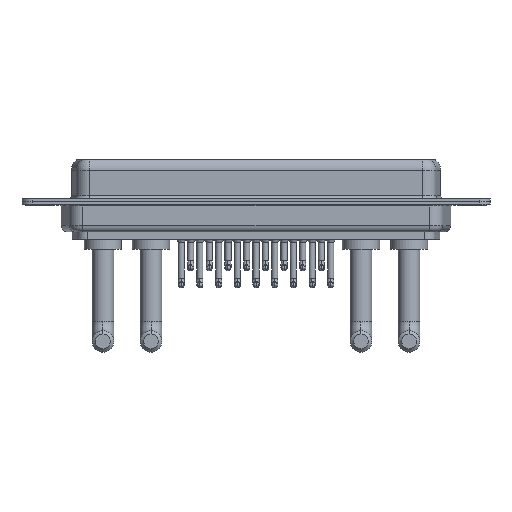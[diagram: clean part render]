
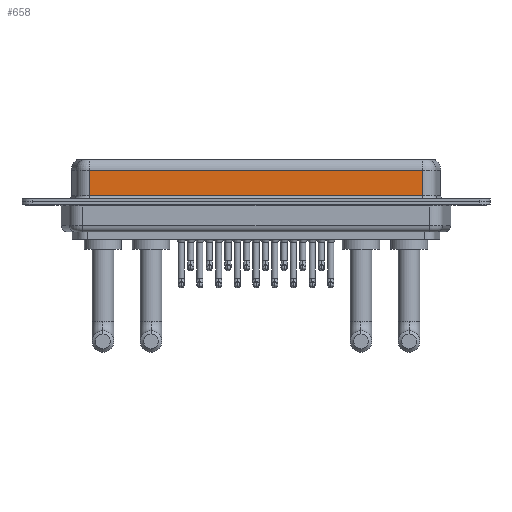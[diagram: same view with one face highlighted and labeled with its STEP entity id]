
A CAD part, front view. The second image highlights one B-rep face of the part: STEP entity #658.
In plain terms, the highlighted planar face has unit normal (0, -1, 0).
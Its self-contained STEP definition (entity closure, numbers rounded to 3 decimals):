
#109 = CARTESIAN_POINT ( 'NONE',  ( 56.462, -3.95, 4.65 ) ) ;
#160 = AXIS2_PLACEMENT_3D ( 'NONE', #12068, #16557, #16660 ) ;
#651 = CARTESIAN_POINT ( 'NONE',  ( 56.462, -3.95, 0.9 ) ) ;
#658 = ADVANCED_FACE ( 'NONE', ( #11863 ), #18094, .F. ) ;
#1508 = CARTESIAN_POINT ( 'NONE',  ( 56.462, -3.95, 6.4 ) ) ;
#2101 = VERTEX_POINT ( 'NONE', #4497 ) ;
#2241 = VECTOR ( 'NONE', #15399, 1000. ) ;
#2499 = EDGE_LOOP ( 'NONE', ( #11322, #4853, #10038, #9736 ) ) ;
#2517 = EDGE_CURVE ( 'NONE', #11364, #8435, #19674, .T. ) ;
#4497 = CARTESIAN_POINT ( 'NONE',  ( 7.038, -3.95, 0.9 ) ) ;
#4853 = ORIENTED_EDGE ( 'NONE', *, *, #2517, .T. ) ;
#5808 = LINE ( 'NONE', #20027, #9830 ) ;
#6004 = DIRECTION ( 'NONE',  ( 0., 0., -1. ) ) ;
#6193 = CARTESIAN_POINT ( 'NONE',  ( 56.462, -3.95, 0.9 ) ) ;
#7419 = CARTESIAN_POINT ( 'NONE',  ( 56.462, -3.95, 4.65 ) ) ;
#8435 = VERTEX_POINT ( 'NONE', #14902 ) ;
#8832 = DIRECTION ( 'NONE',  ( -1., 0., 0. ) ) ;
#9736 = ORIENTED_EDGE ( 'NONE', *, *, #9970, .T. ) ;
#9830 = VECTOR ( 'NONE', #6004, 1000. ) ;
#9970 = EDGE_CURVE ( 'NONE', #2101, #12746, #12141, .T. ) ;
#10038 = ORIENTED_EDGE ( 'NONE', *, *, #12002, .T. ) ;
#11322 = ORIENTED_EDGE ( 'NONE', *, *, #19487, .F. ) ;
#11364 = VERTEX_POINT ( 'NONE', #109 ) ;
#11863 = FACE_OUTER_BOUND ( 'NONE', #2499, .T. ) ;
#12002 = EDGE_CURVE ( 'NONE', #8435, #2101, #5808, .T. ) ;
#12068 = CARTESIAN_POINT ( 'NONE',  ( 56.462, -3.95, 6.4 ) ) ;
#12141 = LINE ( 'NONE', #6193, #2241 ) ;
#12746 = VERTEX_POINT ( 'NONE', #651 ) ;
#14628 = VECTOR ( 'NONE', #8832, 1000. ) ;
#14884 = VECTOR ( 'NONE', #15129, 1000. ) ;
#14902 = CARTESIAN_POINT ( 'NONE',  ( 7.038, -3.95, 4.65 ) ) ;
#15129 = DIRECTION ( 'NONE',  ( 0., 0., -1. ) ) ;
#15399 = DIRECTION ( 'NONE',  ( 1., 0., 0. ) ) ;
#15431 = LINE ( 'NONE', #1508, #14884 ) ;
#16557 = DIRECTION ( 'NONE',  ( 0., 1., 0. ) ) ;
#16660 = DIRECTION ( 'NONE',  ( 0., 0., 1. ) ) ;
#18094 = PLANE ( 'NONE',  #160 ) ;
#19487 = EDGE_CURVE ( 'NONE', #11364, #12746, #15431, .T. ) ;
#19674 = LINE ( 'NONE', #7419, #14628 ) ;
#20027 = CARTESIAN_POINT ( 'NONE',  ( 7.038, -3.95, 6.4 ) ) ;
